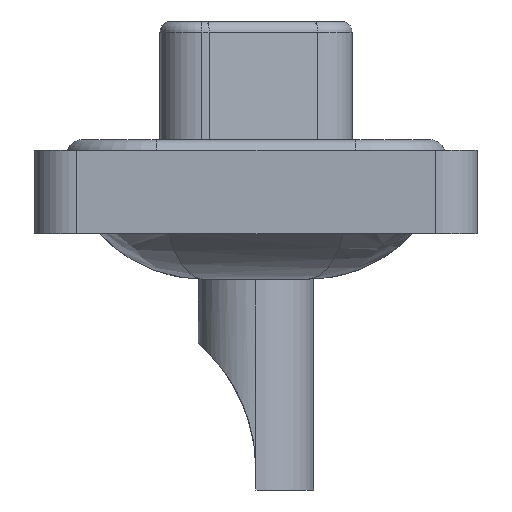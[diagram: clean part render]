
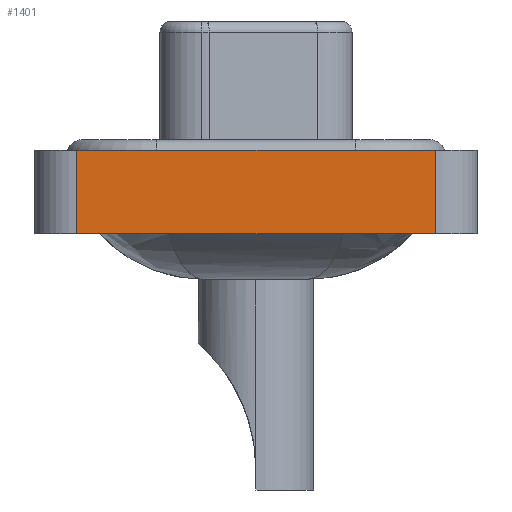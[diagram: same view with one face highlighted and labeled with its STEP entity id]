
A CAD part, left-side view. The second image highlights one B-rep face of the part: STEP entity #1401.
In plain terms, the highlighted planar face has unit normal (-1, 0, 0).
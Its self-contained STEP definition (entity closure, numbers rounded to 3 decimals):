
#304 = DIRECTION ( 'NONE',  ( 0., -1., 0. ) ) ;
#1401 = ADVANCED_FACE ( 'NONE', ( #7641 ), #10666, .T. ) ;
#1503 = VECTOR ( 'NONE', #2488, 1000. ) ;
#1619 = DIRECTION ( 'NONE',  ( 0., -1., 0. ) ) ;
#1703 = LINE ( 'NONE', #9921, #16574 ) ;
#1956 = CARTESIAN_POINT ( 'NONE',  ( -7.35, -8.55, -3.6 ) ) ;
#2488 = DIRECTION ( 'NONE',  ( 0., 0., 1. ) ) ;
#3303 = VECTOR ( 'NONE', #304, 1000. ) ;
#3684 = ORIENTED_EDGE ( 'NONE', *, *, #5517, .F. ) ;
#4721 = CARTESIAN_POINT ( 'NONE',  ( -7.35, -8.55, 0.4 ) ) ;
#5040 = VERTEX_POINT ( 'NONE', #10398 ) ;
#5050 = ORIENTED_EDGE ( 'NONE', *, *, #12145, .T. ) ;
#5306 = EDGE_LOOP ( 'NONE', ( #9377, #10097, #3684, #5050 ) ) ;
#5517 = EDGE_CURVE ( 'NONE', #14886, #5040, #13474, .T. ) ;
#5993 = LINE ( 'NONE', #14229, #3303 ) ;
#7164 = VERTEX_POINT ( 'NONE', #14735 ) ;
#7641 = FACE_OUTER_BOUND ( 'NONE', #5306, .T. ) ;
#9377 = ORIENTED_EDGE ( 'NONE', *, *, #14345, .T. ) ;
#9921 = CARTESIAN_POINT ( 'NONE',  ( -7.35, -8.55, -3.6 ) ) ;
#10097 = ORIENTED_EDGE ( 'NONE', *, *, #15037, .F. ) ;
#10398 = CARTESIAN_POINT ( 'NONE',  ( -7.35, 8.55, 0.4 ) ) ;
#10666 = PLANE ( 'NONE',  #17282 ) ;
#11143 = DIRECTION ( 'NONE',  ( 0., 0., 1. ) ) ;
#11738 = VERTEX_POINT ( 'NONE', #4721 ) ;
#12145 = EDGE_CURVE ( 'NONE', #14886, #7164, #1703, .T. ) ;
#13423 = DIRECTION ( 'NONE',  ( -1., 0., 0. ) ) ;
#13474 = LINE ( 'NONE', #13576, #15835 ) ;
#13516 = CARTESIAN_POINT ( 'NONE',  ( -7.35, -8.55, -3.6 ) ) ;
#13576 = CARTESIAN_POINT ( 'NONE',  ( -7.35, 8.55, -3.6 ) ) ;
#13616 = CARTESIAN_POINT ( 'NONE',  ( -7.35, 8.55, -3.6 ) ) ;
#13691 = DIRECTION ( 'NONE',  ( 0., 0., 1. ) ) ;
#14229 = CARTESIAN_POINT ( 'NONE',  ( -7.35, -8.55, 0.4 ) ) ;
#14345 = EDGE_CURVE ( 'NONE', #7164, #11738, #14382, .T. ) ;
#14382 = LINE ( 'NONE', #1956, #1503 ) ;
#14735 = CARTESIAN_POINT ( 'NONE',  ( -7.35, -8.55, -3.6 ) ) ;
#14886 = VERTEX_POINT ( 'NONE', #13616 ) ;
#15037 = EDGE_CURVE ( 'NONE', #5040, #11738, #5993, .T. ) ;
#15835 = VECTOR ( 'NONE', #11143, 1000. ) ;
#16574 = VECTOR ( 'NONE', #1619, 1000. ) ;
#17282 = AXIS2_PLACEMENT_3D ( 'NONE', #13516, #13423, #13691 ) ;
